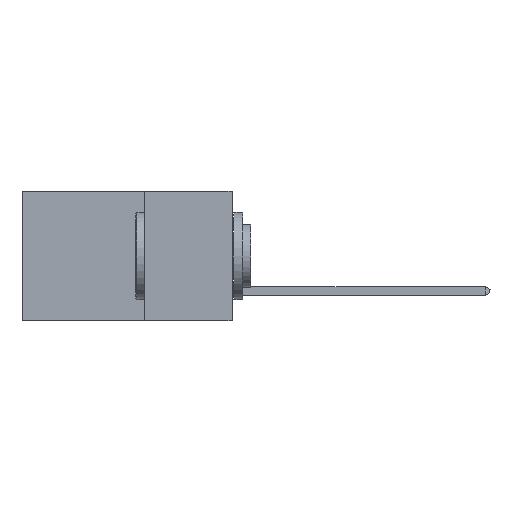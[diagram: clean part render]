
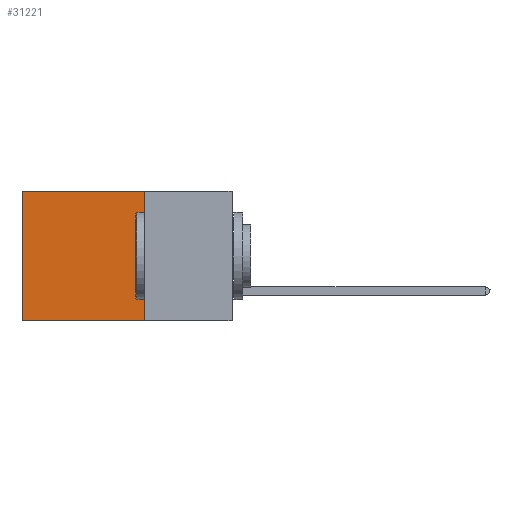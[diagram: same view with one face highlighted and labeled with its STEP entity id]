
A CAD part, left-side view. The second image highlights one B-rep face of the part: STEP entity #31221.
In plain terms, the highlighted planar face has unit normal (-1, 0, 0).
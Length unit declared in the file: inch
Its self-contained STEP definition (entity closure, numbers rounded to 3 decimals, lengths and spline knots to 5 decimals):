
#555 = LINE ( 'NONE', #585, #14128 ) ;
#585 = CARTESIAN_POINT ( 'NONE',  ( 0.2875, 0.25, 0. ) ) ;
#1536 = VECTOR ( 'NONE', #14840, 39.37008 ) ;
#4855 = VERTEX_POINT ( 'NONE', #21150 ) ;
#6537 = ORIENTED_EDGE ( 'NONE', *, *, #40042, .F. ) ;
#6598 = FACE_OUTER_BOUND ( 'NONE', #41196, .T. ) ;
#9189 = PLANE ( 'NONE',  #15178 ) ;
#9202 = CARTESIAN_POINT ( 'NONE',  ( 0.2875, 0.6, 0. ) ) ;
#10940 = LINE ( 'NONE', #9202, #23894 ) ;
#12423 = EDGE_CURVE ( 'NONE', #38168, #4855, #20250, .T. ) ;
#12620 = CARTESIAN_POINT ( 'NONE',  ( 0.2875, 0.25, 0. ) ) ;
#14128 = VECTOR ( 'NONE', #37648, 39.37008 ) ;
#14840 = DIRECTION ( 'NONE',  ( 0., 0., -1. ) ) ;
#15178 = AXIS2_PLACEMENT_3D ( 'NONE', #35843, #17056, #32373 ) ;
#15425 = ORIENTED_EDGE ( 'NONE', *, *, #18297, .T. ) ;
#17056 = DIRECTION ( 'NONE',  ( 1., 0., 0. ) ) ;
#18297 = EDGE_CURVE ( 'NONE', #42140, #29461, #555, .T. ) ;
#20250 = LINE ( 'NONE', #34551, #48012 ) ;
#20344 = LINE ( 'NONE', #33609, #1536 ) ;
#21150 = CARTESIAN_POINT ( 'NONE',  ( 0.2875, 0.6, -0.37 ) ) ;
#22834 = DIRECTION ( 'NONE',  ( 0., 1., 0. ) ) ;
#23894 = VECTOR ( 'NONE', #24137, 39.37008 ) ;
#24137 = DIRECTION ( 'NONE',  ( 0., 0., -1. ) ) ;
#29213 = ORIENTED_EDGE ( 'NONE', *, *, #46056, .T. ) ;
#29461 = VERTEX_POINT ( 'NONE', #39629 ) ;
#31221 = ADVANCED_FACE ( 'NONE', ( #6598 ), #9189, .F. ) ;
#32373 = DIRECTION ( 'NONE',  ( 0., 0., -1. ) ) ;
#33609 = CARTESIAN_POINT ( 'NONE',  ( 0.2875, 0.25, 0. ) ) ;
#34551 = CARTESIAN_POINT ( 'NONE',  ( 0.2875, 0.25, -0.37 ) ) ;
#35843 = CARTESIAN_POINT ( 'NONE',  ( 0.2875, 0.25, 0. ) ) ;
#37648 = DIRECTION ( 'NONE',  ( 0., 1., 0. ) ) ;
#38168 = VERTEX_POINT ( 'NONE', #43679 ) ;
#39064 = ORIENTED_EDGE ( 'NONE', *, *, #12423, .F. ) ;
#39629 = CARTESIAN_POINT ( 'NONE',  ( 0.2875, 0.6, 0. ) ) ;
#40042 = EDGE_CURVE ( 'NONE', #42140, #38168, #20344, .T. ) ;
#41196 = EDGE_LOOP ( 'NONE', ( #29213, #39064, #6537, #15425 ) ) ;
#42140 = VERTEX_POINT ( 'NONE', #12620 ) ;
#43679 = CARTESIAN_POINT ( 'NONE',  ( 0.2875, 0.25, -0.37 ) ) ;
#46056 = EDGE_CURVE ( 'NONE', #29461, #4855, #10940, .T. ) ;
#48012 = VECTOR ( 'NONE', #22834, 39.37008 ) ;
